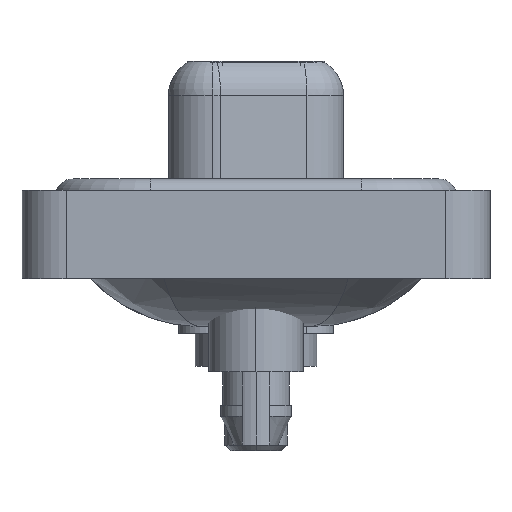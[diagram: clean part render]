
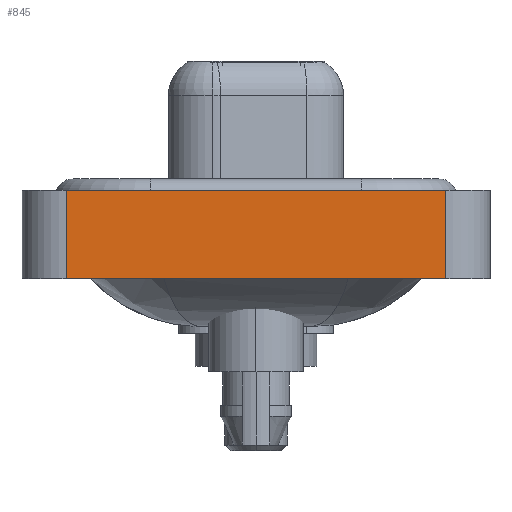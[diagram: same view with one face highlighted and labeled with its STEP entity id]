
A CAD part, left-side view. The second image highlights one B-rep face of the part: STEP entity #845.
In plain terms, the highlighted planar face has unit normal (-1, 0, 0).
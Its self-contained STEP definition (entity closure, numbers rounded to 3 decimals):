
#178 = VERTEX_POINT ( 'NONE', #8979 ) ;
#845 = ADVANCED_FACE ( 'NONE', ( #17203 ), #5004, .T. ) ;
#853 = VERTEX_POINT ( 'NONE', #7734 ) ;
#2094 = VERTEX_POINT ( 'NONE', #6347 ) ;
#2162 = ORIENTED_EDGE ( 'NONE', *, *, #8104, .T. ) ;
#3605 = DIRECTION ( 'NONE',  ( 0., 0., 1. ) ) ;
#4150 = DIRECTION ( 'NONE',  ( 0., 0., 1. ) ) ;
#4435 = CARTESIAN_POINT ( 'NONE',  ( -7.25, 8.55, 0.4 ) ) ;
#4789 = VERTEX_POINT ( 'NONE', #4435 ) ;
#4967 = CARTESIAN_POINT ( 'NONE',  ( -7.25, -8.55, -3.6 ) ) ;
#5004 = PLANE ( 'NONE',  #17124 ) ;
#5080 = EDGE_LOOP ( 'NONE', ( #9062, #11938, #13459, #2162 ) ) ;
#5130 = EDGE_CURVE ( 'NONE', #2094, #178, #11705, .T. ) ;
#5816 = LINE ( 'NONE', #6943, #16248 ) ;
#6347 = CARTESIAN_POINT ( 'NONE',  ( -7.25, -8.55, -3.6 ) ) ;
#6943 = CARTESIAN_POINT ( 'NONE',  ( -7.25, -8.55, -3.6 ) ) ;
#7050 = VECTOR ( 'NONE', #13365, 1000. ) ;
#7734 = CARTESIAN_POINT ( 'NONE',  ( -7.25, 8.55, -3.6 ) ) ;
#8104 = EDGE_CURVE ( 'NONE', #853, #2094, #5816, .T. ) ;
#8979 = CARTESIAN_POINT ( 'NONE',  ( -7.25, -8.55, 0.4 ) ) ;
#9062 = ORIENTED_EDGE ( 'NONE', *, *, #5130, .T. ) ;
#9177 = LINE ( 'NONE', #16983, #7050 ) ;
#9764 = CARTESIAN_POINT ( 'NONE',  ( -7.25, 8.55, -3.6 ) ) ;
#10423 = CARTESIAN_POINT ( 'NONE',  ( -7.25, -8.55, -3.6 ) ) ;
#10725 = VECTOR ( 'NONE', #4150, 1000. ) ;
#10882 = DIRECTION ( 'NONE',  ( 0., -1., 0. ) ) ;
#11400 = VECTOR ( 'NONE', #3605, 1000. ) ;
#11705 = LINE ( 'NONE', #4967, #11400 ) ;
#11938 = ORIENTED_EDGE ( 'NONE', *, *, #13567, .F. ) ;
#13365 = DIRECTION ( 'NONE',  ( 0., -1., 0. ) ) ;
#13459 = ORIENTED_EDGE ( 'NONE', *, *, #16108, .F. ) ;
#13567 = EDGE_CURVE ( 'NONE', #4789, #178, #9177, .T. ) ;
#13675 = LINE ( 'NONE', #9764, #10725 ) ;
#15861 = DIRECTION ( 'NONE',  ( 0., 0., 1. ) ) ;
#16108 = EDGE_CURVE ( 'NONE', #853, #4789, #13675, .T. ) ;
#16248 = VECTOR ( 'NONE', #10882, 1000. ) ;
#16983 = CARTESIAN_POINT ( 'NONE',  ( -7.25, -8.55, 0.4 ) ) ;
#17027 = DIRECTION ( 'NONE',  ( -1., 0., 0. ) ) ;
#17124 = AXIS2_PLACEMENT_3D ( 'NONE', #10423, #17027, #15861 ) ;
#17203 = FACE_OUTER_BOUND ( 'NONE', #5080, .T. ) ;
